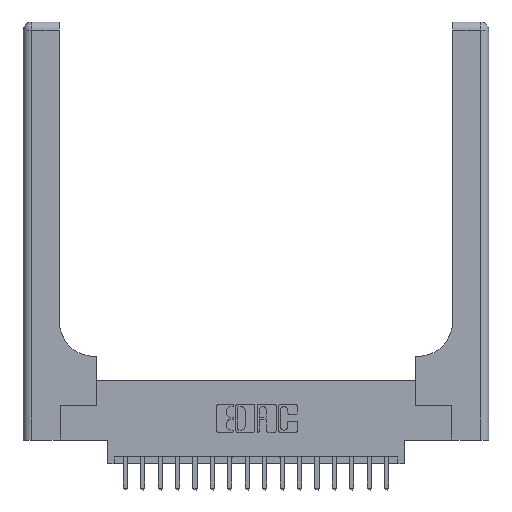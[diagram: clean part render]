
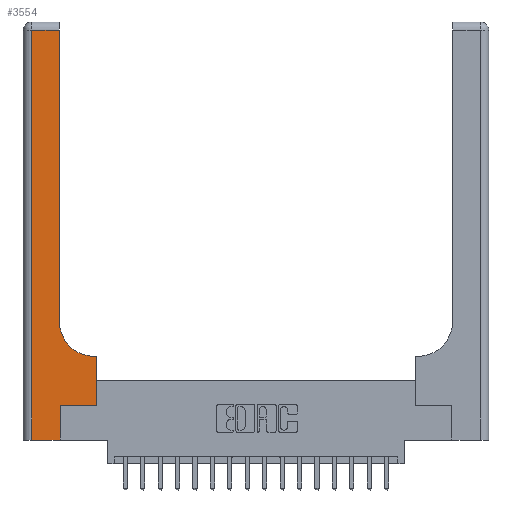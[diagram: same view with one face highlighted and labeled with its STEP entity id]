
A CAD part, top view. The second image highlights one B-rep face of the part: STEP entity #3554.
In plain terms, the highlighted planar face has unit normal (0, 0, 1).
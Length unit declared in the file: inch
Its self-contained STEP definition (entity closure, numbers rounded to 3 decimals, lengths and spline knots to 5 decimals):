
#39 = LINE ( 'NONE', #15479, #5653 ) ;
#41 = CARTESIAN_POINT ( 'NONE',  ( 0.265, 0.25, 0.37 ) ) ;
#133 = CARTESIAN_POINT ( 'NONE',  ( 0.528, 0.6, 0.37 ) ) ;
#138 = LINE ( 'NONE', #41, #16582 ) ;
#684 = VERTEX_POINT ( 'NONE', #16255 ) ;
#705 = DIRECTION ( 'NONE',  ( 0., 0., -1. ) ) ;
#733 = VERTEX_POINT ( 'NONE', #920 ) ;
#816 = CARTESIAN_POINT ( 'NONE',  ( 0., 0., 0.37 ) ) ;
#920 = CARTESIAN_POINT ( 'NONE',  ( 0.26, 0.85, 0.37 ) ) ;
#1004 = EDGE_LOOP ( 'NONE', ( #3056, #17559, #3572, #4775, #16319, #1358, #3307, #10077, #1182 ) ) ;
#1028 = PLANE ( 'NONE',  #8234 ) ;
#1037 = CARTESIAN_POINT ( 'NONE',  ( 0.265, 0., 0.37 ) ) ;
#1182 = ORIENTED_EDGE ( 'NONE', *, *, #3829, .T. ) ;
#1358 = ORIENTED_EDGE ( 'NONE', *, *, #4318, .T. ) ;
#1372 = CARTESIAN_POINT ( 'NONE',  ( 0.06, 0., 0.37 ) ) ;
#1684 = VERTEX_POINT ( 'NONE', #133 ) ;
#1819 = AXIS2_PLACEMENT_3D ( 'NONE', #14246, #705, #12941 ) ;
#2023 = CARTESIAN_POINT ( 'NONE',  ( 0.528, 0.25, 0.37 ) ) ;
#2450 = DIRECTION ( 'NONE',  ( 0., 1., 0. ) ) ;
#2719 = VERTEX_POINT ( 'NONE', #8072 ) ;
#3056 = ORIENTED_EDGE ( 'NONE', *, *, #5316, .T. ) ;
#3096 = EDGE_CURVE ( 'NONE', #16491, #5491, #39, .T. ) ;
#3141 = VECTOR ( 'NONE', #4070, 39.37008 ) ;
#3169 = VECTOR ( 'NONE', #10075, 39.37008 ) ;
#3278 = VECTOR ( 'NONE', #5422, 39.37008 ) ;
#3307 = ORIENTED_EDGE ( 'NONE', *, *, #14885, .T. ) ;
#3518 = LINE ( 'NONE', #816, #3278 ) ;
#3554 = ADVANCED_FACE ( 'NONE', ( #19671 ), #1028, .F. ) ;
#3572 = ORIENTED_EDGE ( 'NONE', *, *, #3096, .T. ) ;
#3829 = EDGE_CURVE ( 'NONE', #2719, #733, #10142, .T. ) ;
#4070 = DIRECTION ( 'NONE',  ( 0., 1., 0. ) ) ;
#4318 = EDGE_CURVE ( 'NONE', #10302, #13909, #138, .T. ) ;
#4775 = ORIENTED_EDGE ( 'NONE', *, *, #12772, .T. ) ;
#5316 = EDGE_CURVE ( 'NONE', #733, #684, #14321, .T. ) ;
#5422 = DIRECTION ( 'NONE',  ( 1., 0., 0. ) ) ;
#5491 = VERTEX_POINT ( 'NONE', #1372 ) ;
#5628 = DIRECTION ( 'NONE',  ( 0., 0., -1. ) ) ;
#5653 = VECTOR ( 'NONE', #10747, 39.37008 ) ;
#5663 = LINE ( 'NONE', #14605, #3169 ) ;
#5930 = DIRECTION ( 'NONE',  ( -1., 0., 0. ) ) ;
#6659 = CARTESIAN_POINT ( 'NONE',  ( 0.06, 2.94, 0.37 ) ) ;
#6681 = VECTOR ( 'NONE', #10064, 39.37008 ) ;
#7138 = CARTESIAN_POINT ( 'NONE',  ( 0., 3., 0.37 ) ) ;
#7674 = VECTOR ( 'NONE', #12559, 39.37008 ) ;
#8039 = CARTESIAN_POINT ( 'NONE',  ( 0., 2.94, 0.37 ) ) ;
#8072 = CARTESIAN_POINT ( 'NONE',  ( 0.51, 0.6, 0.37 ) ) ;
#8099 = EDGE_CURVE ( 'NONE', #8506, #10302, #5663, .T. ) ;
#8234 = AXIS2_PLACEMENT_3D ( 'NONE', #7138, #5628, #5930 ) ;
#8506 = VERTEX_POINT ( 'NONE', #1037 ) ;
#8757 = EDGE_CURVE ( 'NONE', #684, #16491, #18872, .T. ) ;
#10064 = DIRECTION ( 'NONE',  ( -1., 0., 0. ) ) ;
#10075 = DIRECTION ( 'NONE',  ( 0., 1., 0. ) ) ;
#10077 = ORIENTED_EDGE ( 'NONE', *, *, #18920, .T. ) ;
#10142 = CIRCLE ( 'NONE', #1819, 0.25 ) ;
#10287 = CARTESIAN_POINT ( 'NONE',  ( 0.26, 3., 0.37 ) ) ;
#10302 = VERTEX_POINT ( 'NONE', #19068 ) ;
#10747 = DIRECTION ( 'NONE',  ( 0., -1., 0. ) ) ;
#12559 = DIRECTION ( 'NONE',  ( -1., 0., 0. ) ) ;
#12600 = VECTOR ( 'NONE', #2450, 39.37008 ) ;
#12772 = EDGE_CURVE ( 'NONE', #5491, #8506, #3518, .T. ) ;
#12941 = DIRECTION ( 'NONE',  ( 1., 0., 0. ) ) ;
#13909 = VERTEX_POINT ( 'NONE', #2023 ) ;
#14246 = CARTESIAN_POINT ( 'NONE',  ( 0.51, 0.85, 0.37 ) ) ;
#14321 = LINE ( 'NONE', #10287, #3141 ) ;
#14605 = CARTESIAN_POINT ( 'NONE',  ( 0.265, 0., 0.37 ) ) ;
#14691 = LINE ( 'NONE', #17700, #6681 ) ;
#14885 = EDGE_CURVE ( 'NONE', #13909, #1684, #17614, .T. ) ;
#15479 = CARTESIAN_POINT ( 'NONE',  ( 0.06, 3., 0.37 ) ) ;
#16255 = CARTESIAN_POINT ( 'NONE',  ( 0.26, 2.94, 0.37 ) ) ;
#16319 = ORIENTED_EDGE ( 'NONE', *, *, #8099, .T. ) ;
#16491 = VERTEX_POINT ( 'NONE', #6659 ) ;
#16582 = VECTOR ( 'NONE', #16888, 39.37008 ) ;
#16888 = DIRECTION ( 'NONE',  ( 1., 0., 0. ) ) ;
#17513 = CARTESIAN_POINT ( 'NONE',  ( 0.528, 0.25, 0.37 ) ) ;
#17559 = ORIENTED_EDGE ( 'NONE', *, *, #8757, .T. ) ;
#17614 = LINE ( 'NONE', #17513, #12600 ) ;
#17700 = CARTESIAN_POINT ( 'NONE',  ( 0.26, 0.6, 0.37 ) ) ;
#18872 = LINE ( 'NONE', #8039, #7674 ) ;
#18920 = EDGE_CURVE ( 'NONE', #1684, #2719, #14691, .T. ) ;
#19068 = CARTESIAN_POINT ( 'NONE',  ( 0.265, 0.25, 0.37 ) ) ;
#19671 = FACE_OUTER_BOUND ( 'NONE', #1004, .T. ) ;
